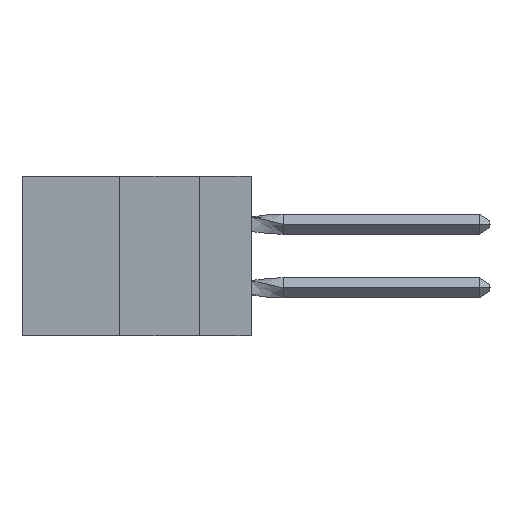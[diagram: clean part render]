
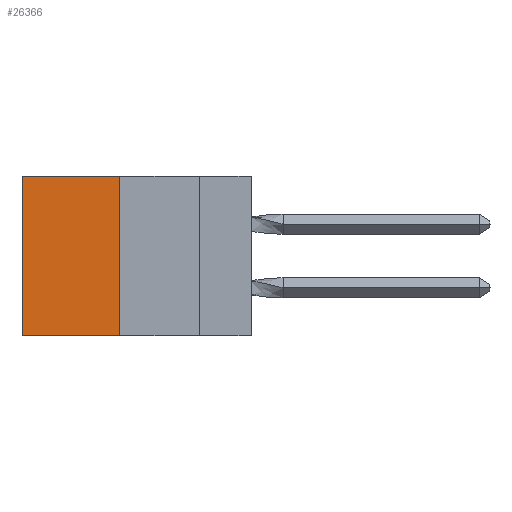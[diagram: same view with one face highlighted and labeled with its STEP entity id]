
A CAD part, left-side view. The second image highlights one B-rep face of the part: STEP entity #26366.
In plain terms, the highlighted planar face has unit normal (-1, 0, 0).
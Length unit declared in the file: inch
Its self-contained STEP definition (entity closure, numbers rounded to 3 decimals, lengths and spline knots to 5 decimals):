
#165 = CARTESIAN_POINT ( 'NONE',  ( 0.305, 0.413, -0.5 ) ) ;
#233 = CARTESIAN_POINT ( 'NONE',  ( 0.305, 0.72, -0.5 ) ) ;
#566 = FACE_OUTER_BOUND ( 'NONE', #21329, .T. ) ;
#2624 = EDGE_CURVE ( 'NONE', #18339, #7014, #2926, .T. ) ;
#2736 = VERTEX_POINT ( 'NONE', #233 ) ;
#2926 = LINE ( 'NONE', #9264, #20367 ) ;
#3251 = CARTESIAN_POINT ( 'NONE',  ( 0.305, 0.72, 0. ) ) ;
#5120 = DIRECTION ( 'NONE',  ( 0., 1., 0. ) ) ;
#5203 = CARTESIAN_POINT ( 'NONE',  ( 0.305, 0.413, 0. ) ) ;
#6242 = DIRECTION ( 'NONE',  ( 0., 0., -1. ) ) ;
#7014 = VERTEX_POINT ( 'NONE', #13747 ) ;
#7042 = VECTOR ( 'NONE', #23621, 39.37008 ) ;
#9264 = CARTESIAN_POINT ( 'NONE',  ( 0.305, 0.413, -0.5 ) ) ;
#11622 = DIRECTION ( 'NONE',  ( 0., 0., -1. ) ) ;
#11764 = EDGE_CURVE ( 'NONE', #7014, #2736, #15613, .T. ) ;
#12070 = CARTESIAN_POINT ( 'NONE',  ( 0.305, 0.413, 0. ) ) ;
#13747 = CARTESIAN_POINT ( 'NONE',  ( 0.305, 0.413, -0.5 ) ) ;
#15613 = LINE ( 'NONE', #25496, #7042 ) ;
#15639 = PLANE ( 'NONE',  #19553 ) ;
#15993 = ORIENTED_EDGE ( 'NONE', *, *, #2624, .F. ) ;
#16453 = ORIENTED_EDGE ( 'NONE', *, *, #22038, .T. ) ;
#16674 = VECTOR ( 'NONE', #6242, 39.37008 ) ;
#17775 = VECTOR ( 'NONE', #5120, 39.37008 ) ;
#18326 = VERTEX_POINT ( 'NONE', #3251 ) ;
#18339 = VERTEX_POINT ( 'NONE', #12070 ) ;
#18584 = EDGE_CURVE ( 'NONE', #18326, #2736, #24188, .T. ) ;
#19553 = AXIS2_PLACEMENT_3D ( 'NONE', #165, #26196, #19642 ) ;
#19642 = DIRECTION ( 'NONE',  ( 0., 0., -1. ) ) ;
#20367 = VECTOR ( 'NONE', #11622, 39.37008 ) ;
#21329 = EDGE_LOOP ( 'NONE', ( #23941, #23950, #15993, #16453 ) ) ;
#22038 = EDGE_CURVE ( 'NONE', #18339, #18326, #23562, .T. ) ;
#23562 = LINE ( 'NONE', #5203, #17775 ) ;
#23621 = DIRECTION ( 'NONE',  ( 0., 1., 0. ) ) ;
#23941 = ORIENTED_EDGE ( 'NONE', *, *, #18584, .T. ) ;
#23950 = ORIENTED_EDGE ( 'NONE', *, *, #11764, .F. ) ;
#24188 = LINE ( 'NONE', #26050, #16674 ) ;
#25496 = CARTESIAN_POINT ( 'NONE',  ( 0.305, 0.413, -0.5 ) ) ;
#26050 = CARTESIAN_POINT ( 'NONE',  ( 0.305, 0.72, -0.5 ) ) ;
#26196 = DIRECTION ( 'NONE',  ( 1., 0., 0. ) ) ;
#26366 = ADVANCED_FACE ( 'NONE', ( #566 ), #15639, .F. ) ;
